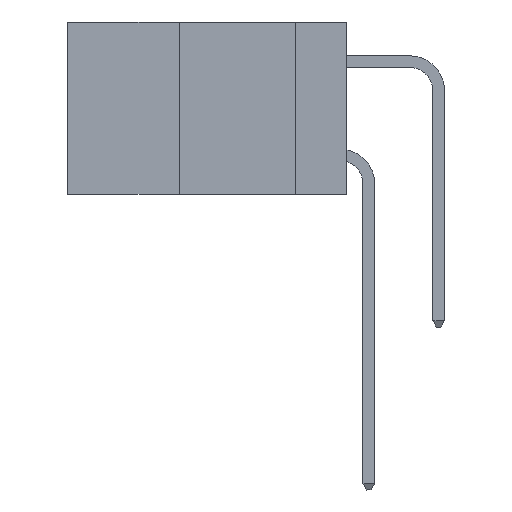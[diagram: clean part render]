
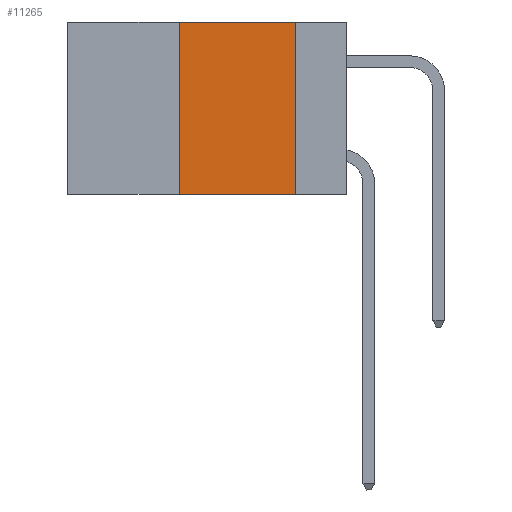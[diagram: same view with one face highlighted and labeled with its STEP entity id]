
A CAD part, left-side view. The second image highlights one B-rep face of the part: STEP entity #11265.
In plain terms, the highlighted planar face has unit normal (-1, 0, 0).
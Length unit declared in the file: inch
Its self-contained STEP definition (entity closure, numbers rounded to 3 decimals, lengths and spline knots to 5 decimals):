
#683 = LINE ( 'NONE', #8371, #11302 ) ;
#1064 = VECTOR ( 'NONE', #8359, 39.37008 ) ;
#1087 = CARTESIAN_POINT ( 'NONE',  ( 0., 0.36, 0. ) ) ;
#1132 = EDGE_CURVE ( 'NONE', #1536, #2859, #11999, .T. ) ;
#1152 = CARTESIAN_POINT ( 'NONE',  ( 0., 0.11, 0. ) ) ;
#1536 = VERTEX_POINT ( 'NONE', #5460 ) ;
#1734 = DIRECTION ( 'NONE',  ( 0., 0., -1. ) ) ;
#1864 = EDGE_LOOP ( 'NONE', ( #11161, #8783, #6333, #3963 ) ) ;
#1914 = VECTOR ( 'NONE', #10479, 39.37008 ) ;
#2859 = VERTEX_POINT ( 'NONE', #1087 ) ;
#3275 = CARTESIAN_POINT ( 'NONE',  ( 0., 0.6, 0. ) ) ;
#3963 = ORIENTED_EDGE ( 'NONE', *, *, #11305, .T. ) ;
#4216 = CARTESIAN_POINT ( 'NONE',  ( 0., 0.11, -0.37 ) ) ;
#5460 = CARTESIAN_POINT ( 'NONE',  ( 0., 0.36, -0.37 ) ) ;
#5851 = PLANE ( 'NONE',  #7585 ) ;
#6053 = VERTEX_POINT ( 'NONE', #1152 ) ;
#6333 = ORIENTED_EDGE ( 'NONE', *, *, #1132, .F. ) ;
#7585 = AXIS2_PLACEMENT_3D ( 'NONE', #9940, #7944, #1734 ) ;
#7869 = EDGE_CURVE ( 'NONE', #2859, #6053, #9513, .T. ) ;
#7944 = DIRECTION ( 'NONE',  ( 1., 0., 0. ) ) ;
#8359 = DIRECTION ( 'NONE',  ( 0., 0., 1. ) ) ;
#8360 = CARTESIAN_POINT ( 'NONE',  ( 0., 0.36, 0. ) ) ;
#8371 = CARTESIAN_POINT ( 'NONE',  ( 0., 0.11, 0. ) ) ;
#8641 = VECTOR ( 'NONE', #11996, 39.37008 ) ;
#8783 = ORIENTED_EDGE ( 'NONE', *, *, #7869, .F. ) ;
#9004 = CARTESIAN_POINT ( 'NONE',  ( 0., 0.6, -0.37 ) ) ;
#9382 = DIRECTION ( 'NONE',  ( 0., 0., -1. ) ) ;
#9513 = LINE ( 'NONE', #3275, #1914 ) ;
#9940 = CARTESIAN_POINT ( 'NONE',  ( 0., 0.6, 0. ) ) ;
#10479 = DIRECTION ( 'NONE',  ( 0., -1., 0. ) ) ;
#11161 = ORIENTED_EDGE ( 'NONE', *, *, #12136, .F. ) ;
#11265 = ADVANCED_FACE ( 'NONE', ( #11635 ), #5851, .F. ) ;
#11302 = VECTOR ( 'NONE', #9382, 39.37008 ) ;
#11305 = EDGE_CURVE ( 'NONE', #1536, #12108, #11328, .T. ) ;
#11328 = LINE ( 'NONE', #9004, #8641 ) ;
#11635 = FACE_OUTER_BOUND ( 'NONE', #1864, .T. ) ;
#11996 = DIRECTION ( 'NONE',  ( 0., -1., 0. ) ) ;
#11999 = LINE ( 'NONE', #8360, #1064 ) ;
#12108 = VERTEX_POINT ( 'NONE', #4216 ) ;
#12136 = EDGE_CURVE ( 'NONE', #6053, #12108, #683, .T. ) ;
